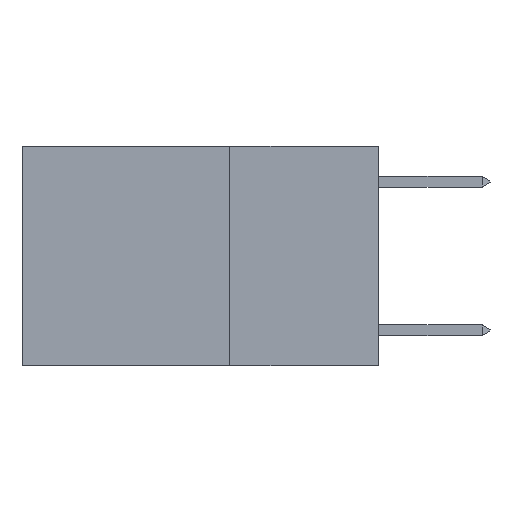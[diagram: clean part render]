
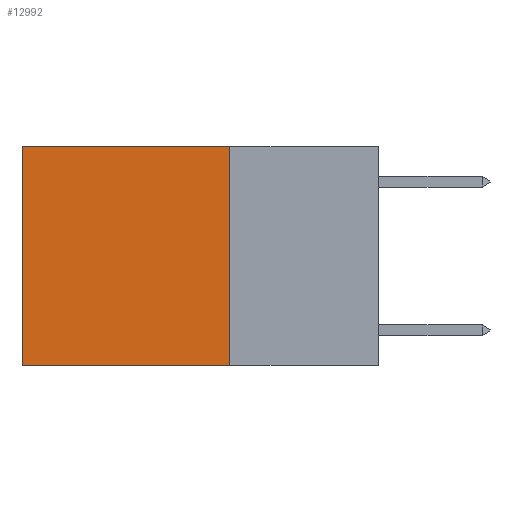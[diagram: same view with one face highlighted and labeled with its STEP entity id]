
A CAD part, left-side view. The second image highlights one B-rep face of the part: STEP entity #12992.
In plain terms, the highlighted planar face has unit normal (-1, 0, 0).
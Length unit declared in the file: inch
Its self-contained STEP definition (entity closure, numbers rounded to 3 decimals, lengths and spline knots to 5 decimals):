
#323 = CARTESIAN_POINT ( 'NONE',  ( 0.2625, 0.25, 0. ) ) ;
#484 = CARTESIAN_POINT ( 'NONE',  ( 0.2625, 0.25, 0. ) ) ;
#648 = DIRECTION ( 'NONE',  ( 1., 0., 0. ) ) ;
#968 = VERTEX_POINT ( 'NONE', #8977 ) ;
#2475 = ORIENTED_EDGE ( 'NONE', *, *, #4980, .T. ) ;
#2924 = LINE ( 'NONE', #3093, #5937 ) ;
#3093 = CARTESIAN_POINT ( 'NONE',  ( 0.2625, 0.25, 0. ) ) ;
#3106 = CARTESIAN_POINT ( 'NONE',  ( 0.2625, 0.25, -0.37 ) ) ;
#3909 = VECTOR ( 'NONE', #12649, 39.37008 ) ;
#4164 = LINE ( 'NONE', #323, #3909 ) ;
#4346 = DIRECTION ( 'NONE',  ( 0., 1., 0. ) ) ;
#4919 = CARTESIAN_POINT ( 'NONE',  ( 0.2625, 0.25, 0. ) ) ;
#4980 = EDGE_CURVE ( 'NONE', #11017, #968, #8660, .T. ) ;
#5087 = DIRECTION ( 'NONE',  ( 0., 0., -1. ) ) ;
#5498 = VERTEX_POINT ( 'NONE', #5768 ) ;
#5748 = ORIENTED_EDGE ( 'NONE', *, *, #6073, .F. ) ;
#5768 = CARTESIAN_POINT ( 'NONE',  ( 0.2625, 0.25, -0.37 ) ) ;
#5937 = VECTOR ( 'NONE', #10113, 39.37008 ) ;
#6070 = EDGE_CURVE ( 'NONE', #13556, #11017, #4164, .T. ) ;
#6073 = EDGE_CURVE ( 'NONE', #13556, #5498, #2924, .T. ) ;
#6326 = CARTESIAN_POINT ( 'NONE',  ( 0.2625, 0.6, 0. ) ) ;
#7949 = ORIENTED_EDGE ( 'NONE', *, *, #6070, .T. ) ;
#8660 = LINE ( 'NONE', #13629, #15768 ) ;
#8977 = CARTESIAN_POINT ( 'NONE',  ( 0.2625, 0.6, -0.37 ) ) ;
#9171 = FACE_OUTER_BOUND ( 'NONE', #15656, .T. ) ;
#10113 = DIRECTION ( 'NONE',  ( 0., 0., -1. ) ) ;
#11017 = VERTEX_POINT ( 'NONE', #6326 ) ;
#11031 = ORIENTED_EDGE ( 'NONE', *, *, #12504, .F. ) ;
#11925 = AXIS2_PLACEMENT_3D ( 'NONE', #484, #648, #14145 ) ;
#12504 = EDGE_CURVE ( 'NONE', #5498, #968, #15461, .T. ) ;
#12649 = DIRECTION ( 'NONE',  ( 0., 1., 0. ) ) ;
#12992 = ADVANCED_FACE ( 'NONE', ( #9171 ), #15442, .F. ) ;
#13556 = VERTEX_POINT ( 'NONE', #4919 ) ;
#13629 = CARTESIAN_POINT ( 'NONE',  ( 0.2625, 0.6, 0. ) ) ;
#14046 = VECTOR ( 'NONE', #4346, 39.37008 ) ;
#14145 = DIRECTION ( 'NONE',  ( 0., 0., -1. ) ) ;
#15442 = PLANE ( 'NONE',  #11925 ) ;
#15461 = LINE ( 'NONE', #3106, #14046 ) ;
#15656 = EDGE_LOOP ( 'NONE', ( #2475, #11031, #5748, #7949 ) ) ;
#15768 = VECTOR ( 'NONE', #5087, 39.37008 ) ;
